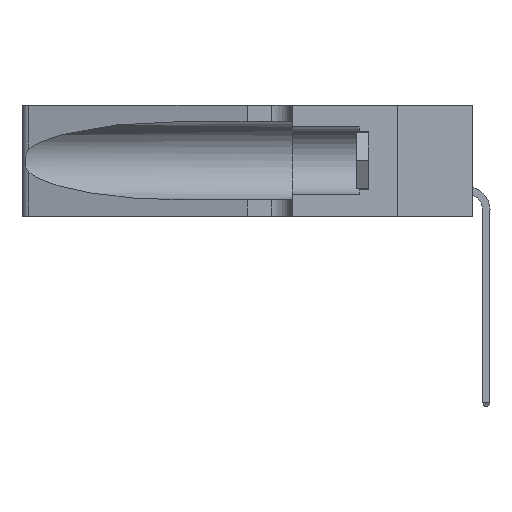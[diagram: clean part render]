
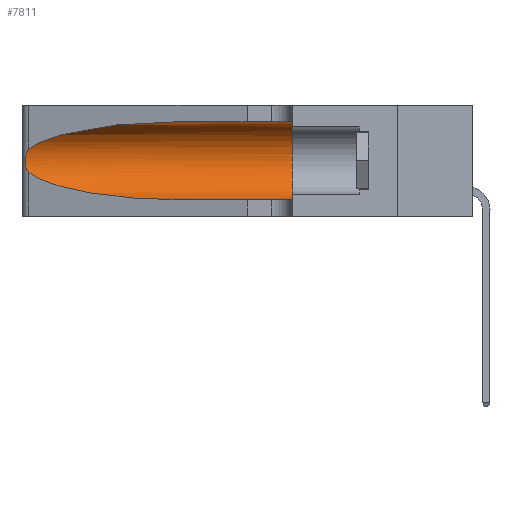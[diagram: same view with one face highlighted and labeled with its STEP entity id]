
A CAD part, left-side view. The second image highlights one B-rep face of the part: STEP entity #7811.
In plain terms, the highlighted cylindrical face has radius 3.308 mm (diameter 6.617 mm), a partial arc.
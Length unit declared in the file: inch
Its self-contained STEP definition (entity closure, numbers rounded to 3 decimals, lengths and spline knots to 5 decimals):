
#182 = ORIENTED_EDGE ( 'NONE', *, *, #3346, .F. ) ;
#245 = CARTESIAN_POINT ( 'NONE',  ( 0.1305, 0.72297, 0.31525 ) ) ;
#699 = AXIS2_PLACEMENT_3D ( 'NONE', #2519, #14913, #2428 ) ;
#1245 = CARTESIAN_POINT ( 'NONE',  ( 0.25787, 1.23484, 0.2124 ) ) ;
#1511 = LINE ( 'NONE', #13842, #25349 ) ;
#1590 = CARTESIAN_POINT ( 'NONE',  ( 0.25639, 1.23186, 0.15144 ) ) ;
#2131 = CARTESIAN_POINT ( 'NONE',  ( 0.1305, 1.61858, 0.31525 ) ) ;
#2153 = VERTEX_POINT ( 'NONE', #3889 ) ;
#2260 = VERTEX_POINT ( 'NONE', #245 ) ;
#2428 = DIRECTION ( 'NONE',  ( 0., 0., 1. ) ) ;
#2519 = CARTESIAN_POINT ( 'NONE',  ( 0.1305, 0.35, 0.185 ) ) ;
#3283 = VERTEX_POINT ( 'NONE', #24963 ) ;
#3346 = EDGE_CURVE ( 'NONE', #2260, #3283, #13374, .T. ) ;
#3424 = CARTESIAN_POINT ( 'NONE',  ( 0.25487, 1.22718, 0.22369 ) ) ;
#3702 = DIRECTION ( 'NONE',  ( 0., -1., 0. ) ) ;
#3889 = CARTESIAN_POINT ( 'NONE',  ( 0.1305, 0.35, 0.05475 ) ) ;
#4574 = CARTESIAN_POINT ( 'NONE',  ( 0.1305, 0.72297, 0.05475 ) ) ;
#5600 = CARTESIAN_POINT ( 'NONE',  ( 0.25789, 1.23486, 0.15765 ) ) ;
#5676 = CARTESIAN_POINT ( 'NONE',  ( 0.25555, 1.22993, 0.14849 ) ) ;
#6318 = CIRCLE ( 'NONE', #699, 0.13025 ) ;
#7191 = CARTESIAN_POINT ( 'NONE',  ( 0.1305, 0.72297, 0.31525 ) ) ;
#7611 = CARTESIAN_POINT ( 'NONE',  ( 0.25487, 1.22718, 0.22369 ) ) ;
#7811 = ADVANCED_FACE ( 'NONE', ( #26628 ), #18115, .F. ) ;
#8151 = EDGE_LOOP ( 'NONE', ( #25296, #24142, #24972, #11045, #17598, #182 ) ) ;
#9601 = CARTESIAN_POINT ( 'NONE',  ( 0.25639, 1.23184, 0.21858 ) ) ;
#9859 = CARTESIAN_POINT ( 'NONE',  ( 0.25856, 1.23593, 0.16098 ) ) ;
#10123 = EDGE_CURVE ( 'NONE', #22858, #19245, #19949, .T. ) ;
#10416 = DIRECTION ( 'NONE',  ( 0., -1., 0. ) ) ;
#10752 = EDGE_CURVE ( 'NONE', #2260, #12153, #26487, .T. ) ;
#11045 = ORIENTED_EDGE ( 'NONE', *, *, #14958, .T. ) ;
#11884 = CARTESIAN_POINT ( 'NONE',  ( 0.26017, 1.23833, 0.17102 ) ) ;
#12153 = VERTEX_POINT ( 'NONE', #19680 ) ;
#12223 = AXIS2_PLACEMENT_3D ( 'NONE', #16130, #3702, #22533 ) ;
#12236 = CARTESIAN_POINT ( 'NONE',  ( 0.1305, 0.72297, 0.05475 ) ) ;
#13374 = LINE ( 'NONE', #2131, #20548 ) ;
#13842 = CARTESIAN_POINT ( 'NONE',  ( 0.1305, 1.61858, 0.05475 ) ) ;
#13995 = CARTESIAN_POINT ( 'NONE',  ( 0.26075, 1.23896, 0.178 ) ) ;
#14913 = DIRECTION ( 'NONE',  ( 0., 1., 0. ) ) ;
#14958 = EDGE_CURVE ( 'NONE', #19245, #2153, #1511, .T. ) ;
#16130 = CARTESIAN_POINT ( 'NONE',  ( 0.1305, 1.61858, 0.185 ) ) ;
#16992 = DIRECTION ( 'NONE',  ( 0., -1., 0. ) ) ;
#17076 = CARTESIAN_POINT ( 'NONE',  ( 0.18966, 0.96281, 0.05475 ) ) ;
#17598 = ORIENTED_EDGE ( 'NONE', *, *, #18047, .F. ) ;
#18047 = EDGE_CURVE ( 'NONE', #3283, #2153, #6318, .T. ) ;
#18115 = CYLINDRICAL_SURFACE ( 'NONE', #12223, 0.13025 ) ;
#18263 = B_SPLINE_CURVE_WITH_KNOTS ( 'NONE', 3,
 ( #7611, #24587, #9601, #1245, #20127, #20297, #22494, #13995, #11884, #9859, #5600, #1590, #5676, #22241 ),
 .UNSPECIFIED., .F., .F.,
 ( 4, 2, 2, 2, 2, 2, 4 ),
 ( 0., 0.00027, 0.00053, 0.00107, 0.0016, 0.00187, 0.00214 ),
 .UNSPECIFIED. ) ;
#19245 = VERTEX_POINT ( 'NONE', #12236 ) ;
#19680 = CARTESIAN_POINT ( 'NONE',  ( 0.25487, 1.22718, 0.22369 ) ) ;
#19949 =( BOUNDED_CURVE ( )  B_SPLINE_CURVE ( 3, ( #25307, #25498, #17076, #4574 ),
 .UNSPECIFIED., .F., .F. ) 
 B_SPLINE_CURVE_WITH_KNOTS ( ( 4, 4 ),
 ( 3.44316, 4.71239 ),
 .UNSPECIFIED. ) 
 CURVE ( )  GEOMETRIC_REPRESENTATION_ITEM ( )  RATIONAL_B_SPLINE_CURVE ( ( 1., 0.87, 0.87, 1. ) ) 
 REPRESENTATION_ITEM ( '' )  );
#20127 = CARTESIAN_POINT ( 'NONE',  ( 0.25854, 1.2359, 0.20912 ) ) ;
#20297 = CARTESIAN_POINT ( 'NONE',  ( 0.26018, 1.23835, 0.19895 ) ) ;
#20548 = VECTOR ( 'NONE', #16992, 39.37008 ) ;
#22180 = CARTESIAN_POINT ( 'NONE',  ( 0.2373, 1.15595, 0.28018 ) ) ;
#22241 = CARTESIAN_POINT ( 'NONE',  ( 0.25487, 1.22718, 0.14631 ) ) ;
#22494 = CARTESIAN_POINT ( 'NONE',  ( 0.26075, 1.23896, 0.19203 ) ) ;
#22533 = DIRECTION ( 'NONE',  ( 0., 0., -1. ) ) ;
#22858 = VERTEX_POINT ( 'NONE', #24714 ) ;
#23321 = EDGE_CURVE ( 'NONE', #12153, #22858, #18263, .T. ) ;
#23715 = CARTESIAN_POINT ( 'NONE',  ( 0.18966, 0.96281, 0.31525 ) ) ;
#24142 = ORIENTED_EDGE ( 'NONE', *, *, #23321, .T. ) ;
#24587 = CARTESIAN_POINT ( 'NONE',  ( 0.25555, 1.22994, 0.2215 ) ) ;
#24714 = CARTESIAN_POINT ( 'NONE',  ( 0.25487, 1.22718, 0.14631 ) ) ;
#24963 = CARTESIAN_POINT ( 'NONE',  ( 0.1305, 0.35, 0.31525 ) ) ;
#24972 = ORIENTED_EDGE ( 'NONE', *, *, #10123, .T. ) ;
#25296 = ORIENTED_EDGE ( 'NONE', *, *, #10752, .T. ) ;
#25307 = CARTESIAN_POINT ( 'NONE',  ( 0.25487, 1.22718, 0.14631 ) ) ;
#25349 = VECTOR ( 'NONE', #10416, 39.37008 ) ;
#25498 = CARTESIAN_POINT ( 'NONE',  ( 0.2373, 1.15595, 0.08982 ) ) ;
#26487 =( BOUNDED_CURVE ( )  B_SPLINE_CURVE ( 3, ( #7191, #23715, #22180, #3424 ),
 .UNSPECIFIED., .F., .F. ) 
 B_SPLINE_CURVE_WITH_KNOTS ( ( 4, 4 ),
 ( 1.5708, 2.84003 ),
 .UNSPECIFIED. ) 
 CURVE ( )  GEOMETRIC_REPRESENTATION_ITEM ( )  RATIONAL_B_SPLINE_CURVE ( ( 1., 0.87, 0.87, 1. ) ) 
 REPRESENTATION_ITEM ( '' )  );
#26628 = FACE_OUTER_BOUND ( 'NONE', #8151, .T. ) ;
